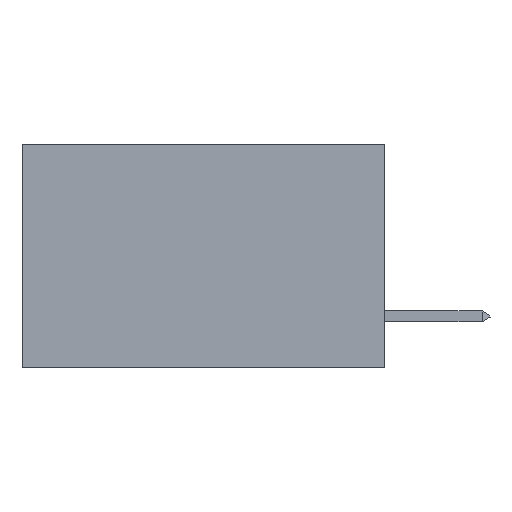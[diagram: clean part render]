
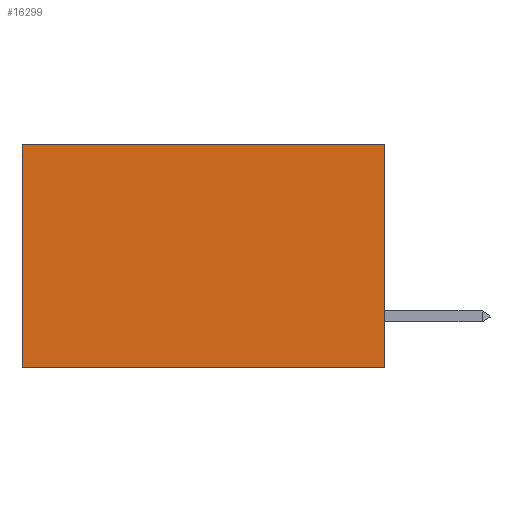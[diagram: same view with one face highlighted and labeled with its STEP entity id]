
A CAD part, left-side view. The second image highlights one B-rep face of the part: STEP entity #16299.
In plain terms, the highlighted planar face has unit normal (-1, 0, 0).
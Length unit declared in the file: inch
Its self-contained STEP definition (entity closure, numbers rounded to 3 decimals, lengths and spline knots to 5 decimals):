
#596 = DIRECTION ( 'NONE',  ( 0., 0., -1. ) ) ;
#822 = CARTESIAN_POINT ( 'NONE',  ( 0.2875, 0., 0. ) ) ;
#1236 = ORIENTED_EDGE ( 'NONE', *, *, #17115, .T. ) ;
#2494 = CARTESIAN_POINT ( 'NONE',  ( 0.2875, 0.6, 0. ) ) ;
#2635 = VECTOR ( 'NONE', #6445, 39.37008 ) ;
#2822 = CARTESIAN_POINT ( 'NONE',  ( 0.2875, 0., 0. ) ) ;
#4938 = CARTESIAN_POINT ( 'NONE',  ( 0.2875, 0., 0. ) ) ;
#5585 = LINE ( 'NONE', #22148, #11579 ) ;
#5806 = VERTEX_POINT ( 'NONE', #11752 ) ;
#6445 = DIRECTION ( 'NONE',  ( 0., 0., -1. ) ) ;
#6570 = DIRECTION ( 'NONE',  ( 0., 0., -1. ) ) ;
#7668 = LINE ( 'NONE', #822, #2635 ) ;
#7987 = CARTESIAN_POINT ( 'NONE',  ( 0.2875, 0., 0. ) ) ;
#10166 = ORIENTED_EDGE ( 'NONE', *, *, #21731, .F. ) ;
#10236 = EDGE_LOOP ( 'NONE', ( #1236, #10166, #13429, #18613 ) ) ;
#10732 = VECTOR ( 'NONE', #6570, 39.37008 ) ;
#10742 = AXIS2_PLACEMENT_3D ( 'NONE', #7987, #12027, #596 ) ;
#11080 = DIRECTION ( 'NONE',  ( 0., 1., 0. ) ) ;
#11226 = VERTEX_POINT ( 'NONE', #2494 ) ;
#11579 = VECTOR ( 'NONE', #11080, 39.37008 ) ;
#11752 = CARTESIAN_POINT ( 'NONE',  ( 0.2875, 0., -0.37 ) ) ;
#11913 = LINE ( 'NONE', #2822, #18473 ) ;
#12027 = DIRECTION ( 'NONE',  ( 1., 0., 0. ) ) ;
#12054 = CARTESIAN_POINT ( 'NONE',  ( 0.2875, 0.6, 0. ) ) ;
#12551 = EDGE_CURVE ( 'NONE', #22587, #5806, #7668, .T. ) ;
#13429 = ORIENTED_EDGE ( 'NONE', *, *, #12551, .F. ) ;
#15745 = VERTEX_POINT ( 'NONE', #20941 ) ;
#16299 = ADVANCED_FACE ( 'NONE', ( #16758 ), #19765, .F. ) ;
#16758 = FACE_OUTER_BOUND ( 'NONE', #10236, .T. ) ;
#17115 = EDGE_CURVE ( 'NONE', #11226, #15745, #22328, .T. ) ;
#17289 = EDGE_CURVE ( 'NONE', #22587, #11226, #11913, .T. ) ;
#18473 = VECTOR ( 'NONE', #23696, 39.37008 ) ;
#18613 = ORIENTED_EDGE ( 'NONE', *, *, #17289, .T. ) ;
#19765 = PLANE ( 'NONE',  #10742 ) ;
#20941 = CARTESIAN_POINT ( 'NONE',  ( 0.2875, 0.6, -0.37 ) ) ;
#21731 = EDGE_CURVE ( 'NONE', #5806, #15745, #5585, .T. ) ;
#22148 = CARTESIAN_POINT ( 'NONE',  ( 0.2875, 0., -0.37 ) ) ;
#22328 = LINE ( 'NONE', #12054, #10732 ) ;
#22587 = VERTEX_POINT ( 'NONE', #4938 ) ;
#23696 = DIRECTION ( 'NONE',  ( 0., 1., 0. ) ) ;
